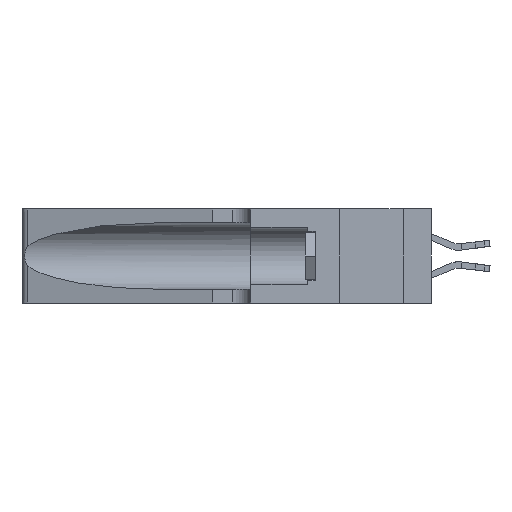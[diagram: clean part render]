
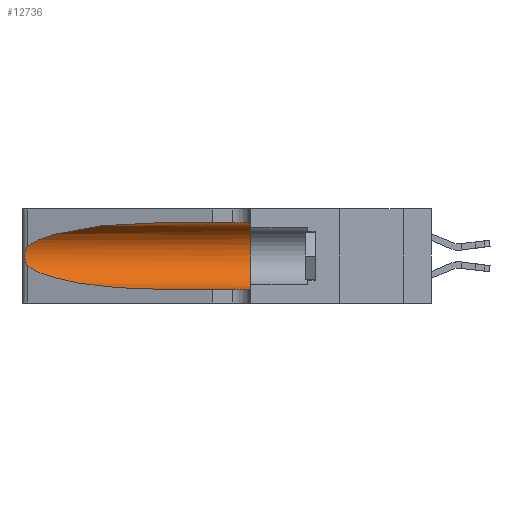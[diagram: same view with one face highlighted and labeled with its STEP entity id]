
A CAD part, left-side view. The second image highlights one B-rep face of the part: STEP entity #12736.
In plain terms, the highlighted cylindrical face has radius 3.308 mm (diameter 6.617 mm), a partial arc.
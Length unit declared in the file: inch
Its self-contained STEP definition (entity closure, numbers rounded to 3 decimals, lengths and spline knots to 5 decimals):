
#425 = CARTESIAN_POINT ( 'NONE',  ( 0.25787, 1.23484, 0.2124 ) ) ;
#1673 = LINE ( 'NONE', #22217, #23657 ) ;
#2726 = CARTESIAN_POINT ( 'NONE',  ( 0.26018, 1.23835, 0.19895 ) ) ;
#2859 = DIRECTION ( 'NONE',  ( 0., -1., 0. ) ) ;
#3878 = EDGE_CURVE ( 'NONE', #21707, #27819, #11242, .T. ) ;
#4069 = EDGE_CURVE ( 'NONE', #20658, #12641, #10326, .T. ) ;
#4727 = ORIENTED_EDGE ( 'NONE', *, *, #10805, .T. ) ;
#4938 = CARTESIAN_POINT ( 'NONE',  ( 0.26075, 1.23896, 0.178 ) ) ;
#5069 = CARTESIAN_POINT ( 'NONE',  ( 0.1305, 0.72297, 0.31525 ) ) ;
#6995 =( BOUNDED_CURVE ( )  B_SPLINE_CURVE ( 3, ( #16583, #9892, #20932, #7784 ),
 .UNSPECIFIED., .F., .F. ) 
 B_SPLINE_CURVE_WITH_KNOTS ( ( 4, 4 ),
 ( 3.44316, 4.71239 ),
 .UNSPECIFIED. ) 
 CURVE ( )  GEOMETRIC_REPRESENTATION_ITEM ( )  RATIONAL_B_SPLINE_CURVE ( ( 1., 0.87, 0.87, 1. ) ) 
 REPRESENTATION_ITEM ( '' )  );
#7178 = CARTESIAN_POINT ( 'NONE',  ( 0.25856, 1.23593, 0.16098 ) ) ;
#7275 = CARTESIAN_POINT ( 'NONE',  ( 0.25487, 1.22718, 0.14631 ) ) ;
#7630 = ORIENTED_EDGE ( 'NONE', *, *, #13313, .T. ) ;
#7784 = CARTESIAN_POINT ( 'NONE',  ( 0.1305, 0.72297, 0.05475 ) ) ;
#9381 = CARTESIAN_POINT ( 'NONE',  ( 0.25639, 1.23186, 0.15144 ) ) ;
#9516 = CARTESIAN_POINT ( 'NONE',  ( 0.18966, 0.96281, 0.31525 ) ) ;
#9892 = CARTESIAN_POINT ( 'NONE',  ( 0.2373, 1.15595, 0.08982 ) ) ;
#10326 = LINE ( 'NONE', #27472, #26988 ) ;
#10376 = FACE_OUTER_BOUND ( 'NONE', #11725, .T. ) ;
#10805 = EDGE_CURVE ( 'NONE', #20658, #21707, #17285, .T. ) ;
#11242 = B_SPLINE_CURVE_WITH_KNOTS ( 'NONE', 3,
 ( #26716, #11514, #24551, #425, #15963, #2726, #18191, #4938, #20346, #7178, #22486, #9381, #24648, #11609 ),
 .UNSPECIFIED., .F., .F.,
 ( 4, 2, 2, 2, 2, 2, 4 ),
 ( 0., 0.00027, 0.00053, 0.00107, 0.0016, 0.00187, 0.00214 ),
 .UNSPECIFIED. ) ;
#11514 = CARTESIAN_POINT ( 'NONE',  ( 0.25555, 1.22994, 0.2215 ) ) ;
#11609 = CARTESIAN_POINT ( 'NONE',  ( 0.25487, 1.22718, 0.14631 ) ) ;
#11725 = EDGE_LOOP ( 'NONE', ( #4727, #21001, #24634, #7630, #28269, #12046 ) ) ;
#11747 = CARTESIAN_POINT ( 'NONE',  ( 0.2373, 1.15595, 0.28018 ) ) ;
#12046 = ORIENTED_EDGE ( 'NONE', *, *, #4069, .F. ) ;
#12243 = CARTESIAN_POINT ( 'NONE',  ( 0.1305, 0.72297, 0.05475 ) ) ;
#12641 = VERTEX_POINT ( 'NONE', #22345 ) ;
#12736 = ADVANCED_FACE ( 'NONE', ( #10376 ), #27039, .F. ) ;
#12917 = CARTESIAN_POINT ( 'NONE',  ( 0.1305, 0.35, 0.185 ) ) ;
#13313 = EDGE_CURVE ( 'NONE', #27288, #25669, #1673, .T. ) ;
#13639 = CARTESIAN_POINT ( 'NONE',  ( 0.25487, 1.22718, 0.22369 ) ) ;
#15140 = DIRECTION ( 'NONE',  ( 0., 0., 1. ) ) ;
#15963 = CARTESIAN_POINT ( 'NONE',  ( 0.25854, 1.2359, 0.20912 ) ) ;
#16106 = DIRECTION ( 'NONE',  ( 0., 0., -1. ) ) ;
#16583 = CARTESIAN_POINT ( 'NONE',  ( 0.25487, 1.22718, 0.14631 ) ) ;
#17285 =( BOUNDED_CURVE ( )  B_SPLINE_CURVE ( 3, ( #5069, #9516, #11747, #26935 ),
 .UNSPECIFIED., .F., .T. ) 
 B_SPLINE_CURVE_WITH_KNOTS ( ( 4, 4 ),
 ( 1.5708, 2.84003 ),
 .UNSPECIFIED. ) 
 CURVE ( )  GEOMETRIC_REPRESENTATION_ITEM ( )  RATIONAL_B_SPLINE_CURVE ( ( 1., 0.87, 0.87, 1. ) ) 
 REPRESENTATION_ITEM ( '' )  );
#17550 = EDGE_CURVE ( 'NONE', #27819, #27288, #6995, .T. ) ;
#18191 = CARTESIAN_POINT ( 'NONE',  ( 0.26075, 1.23896, 0.19203 ) ) ;
#19091 = CARTESIAN_POINT ( 'NONE',  ( 0.1305, 0.72297, 0.31525 ) ) ;
#19142 = EDGE_CURVE ( 'NONE', #12641, #25669, #26697, .T. ) ;
#20346 = CARTESIAN_POINT ( 'NONE',  ( 0.26017, 1.23833, 0.17102 ) ) ;
#20388 = CARTESIAN_POINT ( 'NONE',  ( 0.1305, 1.61858, 0.185 ) ) ;
#20658 = VERTEX_POINT ( 'NONE', #19091 ) ;
#20932 = CARTESIAN_POINT ( 'NONE',  ( 0.18966, 0.96281, 0.05475 ) ) ;
#21001 = ORIENTED_EDGE ( 'NONE', *, *, #3878, .T. ) ;
#21707 = VERTEX_POINT ( 'NONE', #13639 ) ;
#22217 = CARTESIAN_POINT ( 'NONE',  ( 0.1305, 1.61858, 0.05475 ) ) ;
#22328 = AXIS2_PLACEMENT_3D ( 'NONE', #20388, #2859, #16106 ) ;
#22345 = CARTESIAN_POINT ( 'NONE',  ( 0.1305, 0.35, 0.31525 ) ) ;
#22486 = CARTESIAN_POINT ( 'NONE',  ( 0.25789, 1.23486, 0.15765 ) ) ;
#23657 = VECTOR ( 'NONE', #24366, 39.37008 ) ;
#23722 = AXIS2_PLACEMENT_3D ( 'NONE', #12917, #28094, #15140 ) ;
#24366 = DIRECTION ( 'NONE',  ( 0., -1., 0. ) ) ;
#24551 = CARTESIAN_POINT ( 'NONE',  ( 0.25639, 1.23184, 0.21858 ) ) ;
#24634 = ORIENTED_EDGE ( 'NONE', *, *, #17550, .T. ) ;
#24648 = CARTESIAN_POINT ( 'NONE',  ( 0.25555, 1.22993, 0.14849 ) ) ;
#25322 = DIRECTION ( 'NONE',  ( 0., -1., 0. ) ) ;
#25669 = VERTEX_POINT ( 'NONE', #28448 ) ;
#26697 = CIRCLE ( 'NONE', #23722, 0.13025 ) ;
#26716 = CARTESIAN_POINT ( 'NONE',  ( 0.25487, 1.22718, 0.22369 ) ) ;
#26935 = CARTESIAN_POINT ( 'NONE',  ( 0.25487, 1.22718, 0.22369 ) ) ;
#26988 = VECTOR ( 'NONE', #25322, 39.37008 ) ;
#27039 = CYLINDRICAL_SURFACE ( 'NONE', #22328, 0.13025 ) ;
#27288 = VERTEX_POINT ( 'NONE', #12243 ) ;
#27472 = CARTESIAN_POINT ( 'NONE',  ( 0.1305, 1.61858, 0.31525 ) ) ;
#27819 = VERTEX_POINT ( 'NONE', #7275 ) ;
#28094 = DIRECTION ( 'NONE',  ( 0., 1., 0. ) ) ;
#28269 = ORIENTED_EDGE ( 'NONE', *, *, #19142, .F. ) ;
#28448 = CARTESIAN_POINT ( 'NONE',  ( 0.1305, 0.35, 0.05475 ) ) ;
